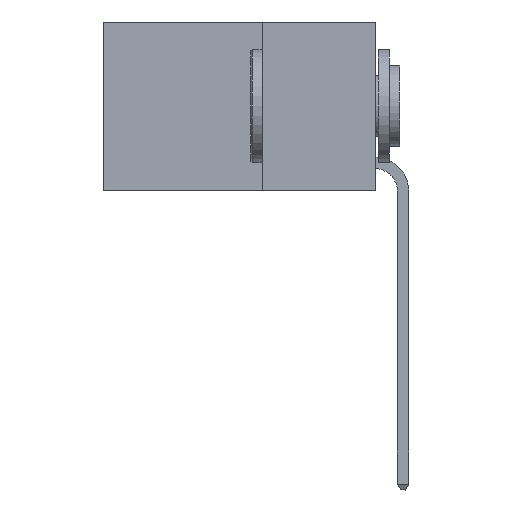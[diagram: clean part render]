
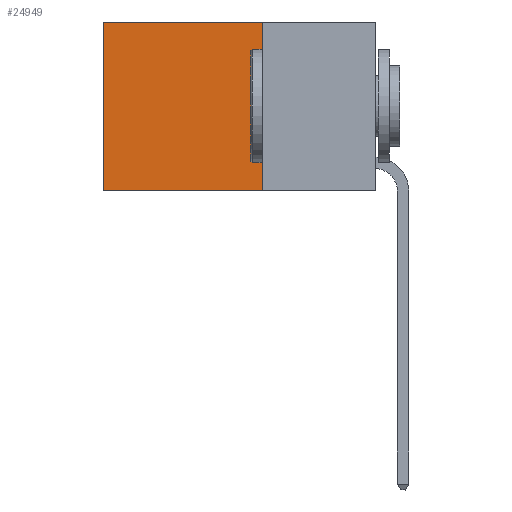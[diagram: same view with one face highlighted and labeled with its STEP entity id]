
A CAD part, left-side view. The second image highlights one B-rep face of the part: STEP entity #24949.
In plain terms, the highlighted planar face has unit normal (-1, 0, 0).
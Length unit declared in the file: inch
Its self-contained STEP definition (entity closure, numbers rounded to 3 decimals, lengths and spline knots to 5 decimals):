
#574 = PLANE ( 'NONE',  #2399 ) ;
#1212 = ORIENTED_EDGE ( 'NONE', *, *, #23120, .T. ) ;
#1538 = CARTESIAN_POINT ( 'NONE',  ( 0.2625, 0.25, -0.37 ) ) ;
#2399 = AXIS2_PLACEMENT_3D ( 'NONE', #16053, #18236, #4986 ) ;
#4986 = DIRECTION ( 'NONE',  ( 0., 0., -1. ) ) ;
#5333 = DIRECTION ( 'NONE',  ( 0., 0., -1. ) ) ;
#5893 = ORIENTED_EDGE ( 'NONE', *, *, #7040, .T. ) ;
#6123 = VERTEX_POINT ( 'NONE', #23335 ) ;
#6165 = ORIENTED_EDGE ( 'NONE', *, *, #19287, .F. ) ;
#6325 = CARTESIAN_POINT ( 'NONE',  ( 0.2625, 0.25, 0. ) ) ;
#7040 = EDGE_CURVE ( 'NONE', #8829, #6123, #22721, .T. ) ;
#7205 = LINE ( 'NONE', #13665, #18281 ) ;
#7980 = DIRECTION ( 'NONE',  ( 0., 1., 0. ) ) ;
#8104 = VERTEX_POINT ( 'NONE', #6325 ) ;
#8829 = VERTEX_POINT ( 'NONE', #17714 ) ;
#13665 = CARTESIAN_POINT ( 'NONE',  ( 0.2625, 0.25, 0. ) ) ;
#15507 = DIRECTION ( 'NONE',  ( 0., 0., -1. ) ) ;
#16053 = CARTESIAN_POINT ( 'NONE',  ( 0.2625, 0.25, 0. ) ) ;
#16141 = ORIENTED_EDGE ( 'NONE', *, *, #18454, .F. ) ;
#16392 = CARTESIAN_POINT ( 'NONE',  ( 0.2625, 0.25, 0. ) ) ;
#17714 = CARTESIAN_POINT ( 'NONE',  ( 0.2625, 0.6, 0. ) ) ;
#18064 = DIRECTION ( 'NONE',  ( 0., 1., 0. ) ) ;
#18236 = DIRECTION ( 'NONE',  ( 1., 0., 0. ) ) ;
#18281 = VECTOR ( 'NONE', #18064, 39.37008 ) ;
#18454 = EDGE_CURVE ( 'NONE', #8104, #26436, #26253, .T. ) ;
#18830 = CARTESIAN_POINT ( 'NONE',  ( 0.2625, 0.25, -0.37 ) ) ;
#19287 = EDGE_CURVE ( 'NONE', #26436, #6123, #28190, .T. ) ;
#21243 = FACE_OUTER_BOUND ( 'NONE', #26195, .T. ) ;
#21248 = VECTOR ( 'NONE', #5333, 39.37008 ) ;
#21969 = CARTESIAN_POINT ( 'NONE',  ( 0.2625, 0.6, 0. ) ) ;
#22062 = VECTOR ( 'NONE', #15507, 39.37008 ) ;
#22721 = LINE ( 'NONE', #21969, #22062 ) ;
#23120 = EDGE_CURVE ( 'NONE', #8104, #8829, #7205, .T. ) ;
#23335 = CARTESIAN_POINT ( 'NONE',  ( 0.2625, 0.6, -0.37 ) ) ;
#24949 = ADVANCED_FACE ( 'NONE', ( #21243 ), #574, .F. ) ;
#26195 = EDGE_LOOP ( 'NONE', ( #5893, #6165, #16141, #1212 ) ) ;
#26253 = LINE ( 'NONE', #16392, #21248 ) ;
#26436 = VERTEX_POINT ( 'NONE', #18830 ) ;
#27523 = VECTOR ( 'NONE', #7980, 39.37008 ) ;
#28190 = LINE ( 'NONE', #1538, #27523 ) ;
